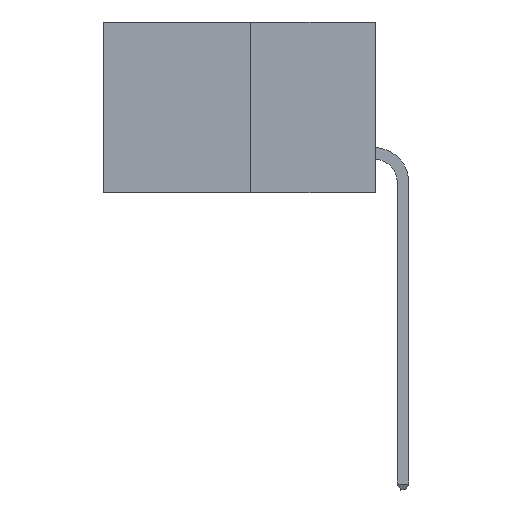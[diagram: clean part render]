
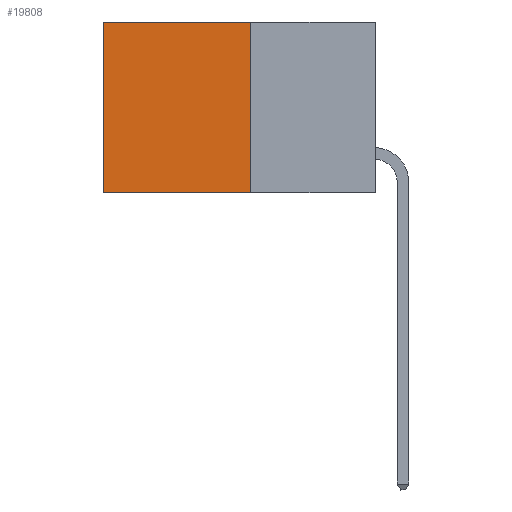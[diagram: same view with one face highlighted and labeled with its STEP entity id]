
A CAD part, left-side view. The second image highlights one B-rep face of the part: STEP entity #19808.
In plain terms, the highlighted planar face has unit normal (-1, 0, 0).
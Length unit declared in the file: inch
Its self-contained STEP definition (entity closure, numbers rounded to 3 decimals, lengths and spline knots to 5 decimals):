
#225 = ORIENTED_EDGE ( 'NONE', *, *, #4966, .F. ) ;
#483 = DIRECTION ( 'NONE',  ( 0., 1., 0. ) ) ;
#532 = DIRECTION ( 'NONE',  ( 0., 1., 0. ) ) ;
#1028 = CARTESIAN_POINT ( 'NONE',  ( 0.277, 0.59, 0. ) ) ;
#1032 = PLANE ( 'NONE',  #17220 ) ;
#1647 = VERTEX_POINT ( 'NONE', #19556 ) ;
#1776 = ORIENTED_EDGE ( 'NONE', *, *, #6204, .F. ) ;
#1964 = VERTEX_POINT ( 'NONE', #19912 ) ;
#2702 = DIRECTION ( 'NONE',  ( 1., 0., 0. ) ) ;
#2775 = VERTEX_POINT ( 'NONE', #11336 ) ;
#3579 = VECTOR ( 'NONE', #483, 39.37008 ) ;
#4052 = CARTESIAN_POINT ( 'NONE',  ( 0.277, 0.27, -0.37 ) ) ;
#4966 = EDGE_CURVE ( 'NONE', #1647, #1964, #7899, .T. ) ;
#5442 = CARTESIAN_POINT ( 'NONE',  ( 0.277, 0.27, 0. ) ) ;
#5668 = VECTOR ( 'NONE', #12651, 39.37008 ) ;
#5789 = CARTESIAN_POINT ( 'NONE',  ( 0.277, 0.27, -0.37 ) ) ;
#5932 = CARTESIAN_POINT ( 'NONE',  ( 0.277, 0.27, -0.37 ) ) ;
#6204 = EDGE_CURVE ( 'NONE', #1964, #2775, #11609, .T. ) ;
#7314 = EDGE_LOOP ( 'NONE', ( #16568, #1776, #225, #10660 ) ) ;
#7411 = VECTOR ( 'NONE', #17797, 39.37008 ) ;
#7899 = LINE ( 'NONE', #4052, #7411 ) ;
#8272 = VECTOR ( 'NONE', #532, 39.37008 ) ;
#8761 = LINE ( 'NONE', #5442, #8272 ) ;
#10404 = VERTEX_POINT ( 'NONE', #1028 ) ;
#10660 = ORIENTED_EDGE ( 'NONE', *, *, #19595, .T. ) ;
#11336 = CARTESIAN_POINT ( 'NONE',  ( 0.277, 0.59, -0.37 ) ) ;
#11609 = LINE ( 'NONE', #5789, #3579 ) ;
#12651 = DIRECTION ( 'NONE',  ( 0., 0., -1. ) ) ;
#13903 = DIRECTION ( 'NONE',  ( 0., 0., -1. ) ) ;
#16568 = ORIENTED_EDGE ( 'NONE', *, *, #16761, .T. ) ;
#16761 = EDGE_CURVE ( 'NONE', #10404, #2775, #18333, .T. ) ;
#17220 = AXIS2_PLACEMENT_3D ( 'NONE', #5932, #2702, #13903 ) ;
#17797 = DIRECTION ( 'NONE',  ( 0., 0., -1. ) ) ;
#18333 = LINE ( 'NONE', #18966, #5668 ) ;
#18959 = FACE_OUTER_BOUND ( 'NONE', #7314, .T. ) ;
#18966 = CARTESIAN_POINT ( 'NONE',  ( 0.277, 0.59, -0.37 ) ) ;
#19556 = CARTESIAN_POINT ( 'NONE',  ( 0.277, 0.27, 0. ) ) ;
#19595 = EDGE_CURVE ( 'NONE', #1647, #10404, #8761, .T. ) ;
#19808 = ADVANCED_FACE ( 'NONE', ( #18959 ), #1032, .F. ) ;
#19912 = CARTESIAN_POINT ( 'NONE',  ( 0.277, 0.27, -0.37 ) ) ;
